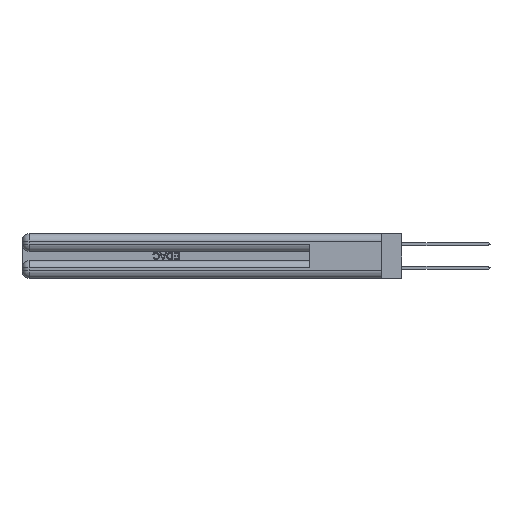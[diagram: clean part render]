
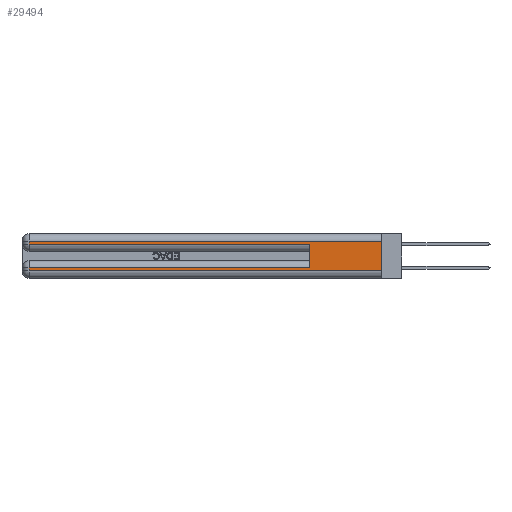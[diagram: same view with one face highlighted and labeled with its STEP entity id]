
A CAD part, left-side view. The second image highlights one B-rep face of the part: STEP entity #29494.
In plain terms, the highlighted planar face has unit normal (-1, 0, 0).
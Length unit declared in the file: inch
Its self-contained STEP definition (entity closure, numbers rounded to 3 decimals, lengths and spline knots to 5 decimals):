
#505 = CARTESIAN_POINT ( 'NONE',  ( 0., 0., 0.06 ) ) ;
#1745 = VERTEX_POINT ( 'NONE', #15747 ) ;
#1784 = ORIENTED_EDGE ( 'NONE', *, *, #16431, .T. ) ;
#1864 = DIRECTION ( 'NONE',  ( 0., 0., -1. ) ) ;
#2132 = CARTESIAN_POINT ( 'NONE',  ( 0., 2.94, 0.085 ) ) ;
#2536 = DIRECTION ( 'NONE',  ( 0., -1., 0. ) ) ;
#2604 = FACE_OUTER_BOUND ( 'NONE', #43405, .T. ) ;
#2878 = DIRECTION ( 'NONE',  ( 0., 1., 0. ) ) ;
#3282 = EDGE_CURVE ( 'NONE', #17421, #30804, #43582, .T. ) ;
#3420 = EDGE_CURVE ( 'NONE', #38326, #11041, #39283, .T. ) ;
#5215 = DIRECTION ( 'NONE',  ( 1., 0., 0. ) ) ;
#5244 = LINE ( 'NONE', #16099, #31322 ) ;
#7632 = VERTEX_POINT ( 'NONE', #39713 ) ;
#8444 = VECTOR ( 'NONE', #8716, 39.37008 ) ;
#8620 = CARTESIAN_POINT ( 'NONE',  ( 0., 2.94, 0.37 ) ) ;
#8716 = DIRECTION ( 'NONE',  ( 0., 1., 0. ) ) ;
#8823 = VECTOR ( 'NONE', #2878, 39.37008 ) ;
#9025 = ORIENTED_EDGE ( 'NONE', *, *, #30181, .T. ) ;
#9785 = CARTESIAN_POINT ( 'NONE',  ( 0., 0., 0.31 ) ) ;
#9953 = ORIENTED_EDGE ( 'NONE', *, *, #11814, .F. ) ;
#11006 = ORIENTED_EDGE ( 'NONE', *, *, #28214, .T. ) ;
#11041 = VERTEX_POINT ( 'NONE', #24723 ) ;
#11814 = EDGE_CURVE ( 'NONE', #17421, #11041, #29217, .T. ) ;
#11883 = DIRECTION ( 'NONE',  ( 0., 0., 1. ) ) ;
#12045 = LINE ( 'NONE', #39766, #29063 ) ;
#15368 = PLANE ( 'NONE',  #43477 ) ;
#15747 = CARTESIAN_POINT ( 'NONE',  ( 0., 2.94, 0.31 ) ) ;
#15981 = VERTEX_POINT ( 'NONE', #505 ) ;
#16099 = CARTESIAN_POINT ( 'NONE',  ( 0., 2.94, 0.37 ) ) ;
#16431 = EDGE_CURVE ( 'NONE', #7632, #1745, #26906, .T. ) ;
#17421 = VERTEX_POINT ( 'NONE', #24564 ) ;
#17694 = CARTESIAN_POINT ( 'NONE',  ( 0., 2.94, 0.285 ) ) ;
#19079 = VECTOR ( 'NONE', #2536, 39.37008 ) ;
#20883 = LINE ( 'NONE', #8620, #37889 ) ;
#21333 = LINE ( 'NONE', #37200, #37285 ) ;
#21931 = ORIENTED_EDGE ( 'NONE', *, *, #3420, .T. ) ;
#22812 = DIRECTION ( 'NONE',  ( 0., -1., 0. ) ) ;
#24564 = CARTESIAN_POINT ( 'NONE',  ( 0., 0.6, 0.085 ) ) ;
#24723 = CARTESIAN_POINT ( 'NONE',  ( 0., 0.6, 0.285 ) ) ;
#25170 = EDGE_CURVE ( 'NONE', #40935, #15981, #12045, .T. ) ;
#25595 = CARTESIAN_POINT ( 'NONE',  ( 0., 0., 0.37 ) ) ;
#25785 = ORIENTED_EDGE ( 'NONE', *, *, #3282, .T. ) ;
#26233 = ORIENTED_EDGE ( 'NONE', *, *, #31709, .F. ) ;
#26906 = LINE ( 'NONE', #9785, #8823 ) ;
#27441 = ORIENTED_EDGE ( 'NONE', *, *, #25170, .T. ) ;
#28214 = EDGE_CURVE ( 'NONE', #30804, #40935, #20883, .T. ) ;
#29043 = DIRECTION ( 'NONE',  ( 0., 0., -1. ) ) ;
#29063 = VECTOR ( 'NONE', #22812, 39.37008 ) ;
#29084 = CARTESIAN_POINT ( 'NONE',  ( 0., 0., 0.085 ) ) ;
#29217 = LINE ( 'NONE', #35647, #33616 ) ;
#29494 = ADVANCED_FACE ( 'NONE', ( #2604 ), #15368, .F. ) ;
#30181 = EDGE_CURVE ( 'NONE', #1745, #38326, #5244, .T. ) ;
#30804 = VERTEX_POINT ( 'NONE', #2132 ) ;
#31322 = VECTOR ( 'NONE', #36431, 39.37008 ) ;
#31530 = CARTESIAN_POINT ( 'NONE',  ( 0., 2.94, 0.06 ) ) ;
#31709 = EDGE_CURVE ( 'NONE', #7632, #15981, #21333, .T. ) ;
#33616 = VECTOR ( 'NONE', #11883, 39.37008 ) ;
#35647 = CARTESIAN_POINT ( 'NONE',  ( 0., 0.6, 0.145 ) ) ;
#36431 = DIRECTION ( 'NONE',  ( 0., 0., -1. ) ) ;
#37200 = CARTESIAN_POINT ( 'NONE',  ( 0., 0., 0.37 ) ) ;
#37285 = VECTOR ( 'NONE', #44068, 39.37008 ) ;
#37889 = VECTOR ( 'NONE', #1864, 39.37008 ) ;
#38326 = VERTEX_POINT ( 'NONE', #17694 ) ;
#39283 = LINE ( 'NONE', #43366, #19079 ) ;
#39713 = CARTESIAN_POINT ( 'NONE',  ( 0., 0., 0.31 ) ) ;
#39766 = CARTESIAN_POINT ( 'NONE',  ( 0., 0., 0.06 ) ) ;
#40935 = VERTEX_POINT ( 'NONE', #31530 ) ;
#43366 = CARTESIAN_POINT ( 'NONE',  ( 0., 0., 0.285 ) ) ;
#43405 = EDGE_LOOP ( 'NONE', ( #26233, #1784, #9025, #21931, #9953, #25785, #11006, #27441 ) ) ;
#43477 = AXIS2_PLACEMENT_3D ( 'NONE', #25595, #5215, #29043 ) ;
#43582 = LINE ( 'NONE', #29084, #8444 ) ;
#44068 = DIRECTION ( 'NONE',  ( 0., 0., -1. ) ) ;
